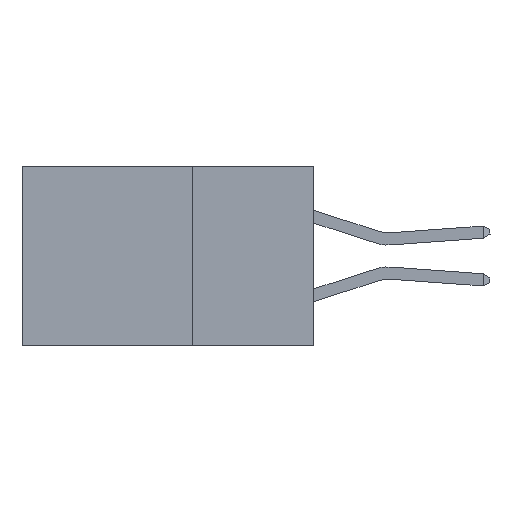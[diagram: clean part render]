
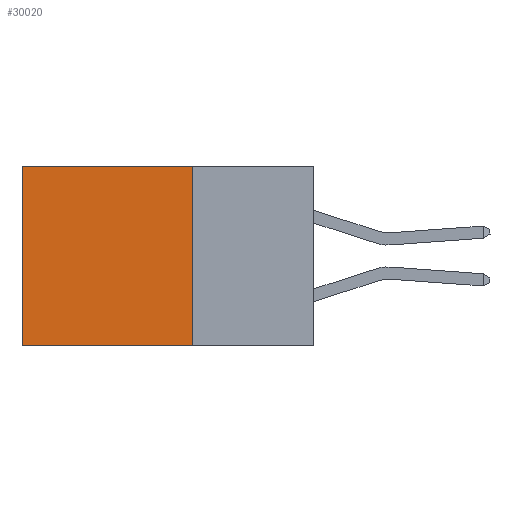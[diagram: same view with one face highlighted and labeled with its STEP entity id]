
A CAD part, left-side view. The second image highlights one B-rep face of the part: STEP entity #30020.
In plain terms, the highlighted planar face has unit normal (-1, 0, 0).
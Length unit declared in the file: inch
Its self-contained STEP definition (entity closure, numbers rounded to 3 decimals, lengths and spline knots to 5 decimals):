
#230 = EDGE_CURVE ( 'NONE', #25509, #15400, #16994, .T. ) ;
#890 = ORIENTED_EDGE ( 'NONE', *, *, #230, .T. ) ;
#1034 = EDGE_CURVE ( 'NONE', #14106, #15400, #38770, .T. ) ;
#1102 = AXIS2_PLACEMENT_3D ( 'NONE', #32822, #14367, #26729 ) ;
#4102 = VECTOR ( 'NONE', #5339, 39.37008 ) ;
#4334 = VECTOR ( 'NONE', #30612, 39.37008 ) ;
#5339 = DIRECTION ( 'NONE',  ( 0., 1., 0. ) ) ;
#7308 = VECTOR ( 'NONE', #23684, 39.37008 ) ;
#8741 = LINE ( 'NONE', #33845, #19550 ) ;
#11131 = PLANE ( 'NONE',  #1102 ) ;
#14106 = VERTEX_POINT ( 'NONE', #38235 ) ;
#14367 = DIRECTION ( 'NONE',  ( 1., 0., 0. ) ) ;
#15400 = VERTEX_POINT ( 'NONE', #26247 ) ;
#15622 = CARTESIAN_POINT ( 'NONE',  ( 0.2875, 0.25, 0. ) ) ;
#16994 = LINE ( 'NONE', #38912, #7308 ) ;
#17651 = CARTESIAN_POINT ( 'NONE',  ( 0.2875, 0.6, 0. ) ) ;
#19074 = ORIENTED_EDGE ( 'NONE', *, *, #1034, .F. ) ;
#19550 = VECTOR ( 'NONE', #30591, 39.37008 ) ;
#20245 = FACE_OUTER_BOUND ( 'NONE', #27156, .T. ) ;
#20277 = ORIENTED_EDGE ( 'NONE', *, *, #39527, .T. ) ;
#23531 = CARTESIAN_POINT ( 'NONE',  ( 0.2875, 0.25, -0.37 ) ) ;
#23684 = DIRECTION ( 'NONE',  ( 0., 0., -1. ) ) ;
#25509 = VERTEX_POINT ( 'NONE', #17651 ) ;
#25655 = EDGE_CURVE ( 'NONE', #34697, #14106, #33870, .T. ) ;
#26247 = CARTESIAN_POINT ( 'NONE',  ( 0.2875, 0.6, -0.37 ) ) ;
#26729 = DIRECTION ( 'NONE',  ( 0., 0., -1. ) ) ;
#27156 = EDGE_LOOP ( 'NONE', ( #890, #19074, #30052, #20277 ) ) ;
#27324 = CARTESIAN_POINT ( 'NONE',  ( 0.2875, 0.25, 0. ) ) ;
#30020 = ADVANCED_FACE ( 'NONE', ( #20245 ), #11131, .F. ) ;
#30052 = ORIENTED_EDGE ( 'NONE', *, *, #25655, .F. ) ;
#30591 = DIRECTION ( 'NONE',  ( 0., 1., 0. ) ) ;
#30612 = DIRECTION ( 'NONE',  ( 0., 0., -1. ) ) ;
#32822 = CARTESIAN_POINT ( 'NONE',  ( 0.2875, 0.25, 0. ) ) ;
#33845 = CARTESIAN_POINT ( 'NONE',  ( 0.2875, 0.25, 0. ) ) ;
#33870 = LINE ( 'NONE', #15622, #4334 ) ;
#34697 = VERTEX_POINT ( 'NONE', #27324 ) ;
#38235 = CARTESIAN_POINT ( 'NONE',  ( 0.2875, 0.25, -0.37 ) ) ;
#38770 = LINE ( 'NONE', #23531, #4102 ) ;
#38912 = CARTESIAN_POINT ( 'NONE',  ( 0.2875, 0.6, 0. ) ) ;
#39527 = EDGE_CURVE ( 'NONE', #34697, #25509, #8741, .T. ) ;
